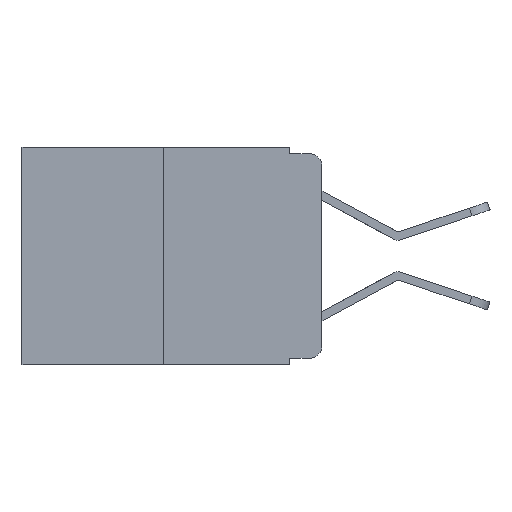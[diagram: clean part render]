
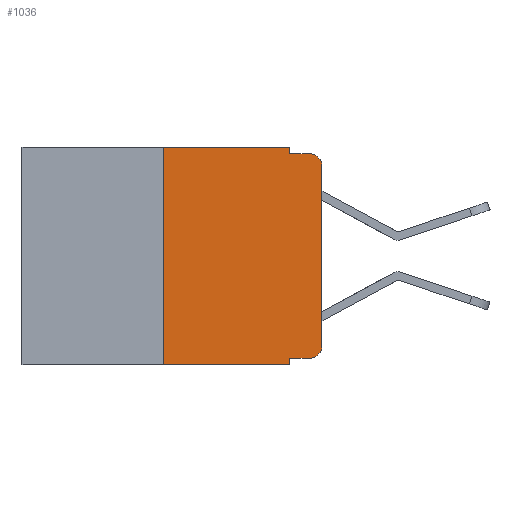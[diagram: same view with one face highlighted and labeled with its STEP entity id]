
A CAD part, left-side view. The second image highlights one B-rep face of the part: STEP entity #1036.
In plain terms, the highlighted planar face has unit normal (-1, 0, 0).
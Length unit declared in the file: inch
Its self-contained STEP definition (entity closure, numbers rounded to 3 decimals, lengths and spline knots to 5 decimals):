
#173 = VECTOR ( 'NONE', #9274, 39.37008 ) ;
#390 = DIRECTION ( 'NONE',  ( 0., 0., 1. ) ) ;
#671 = ORIENTED_EDGE ( 'NONE', *, *, #6945, .F. ) ;
#706 = ORIENTED_EDGE ( 'NONE', *, *, #1145, .T. ) ;
#812 = VERTEX_POINT ( 'NONE', #8968 ) ;
#838 = VECTOR ( 'NONE', #9036, 39.37008 ) ;
#891 = AXIS2_PLACEMENT_3D ( 'NONE', #4014, #6603, #8453 ) ;
#997 = EDGE_CURVE ( 'NONE', #5540, #1076, #4803, .T. ) ;
#1036 = ADVANCED_FACE ( 'NONE', ( #9545 ), #1417, .F. ) ;
#1076 = VERTEX_POINT ( 'NONE', #3899 ) ;
#1145 = EDGE_CURVE ( 'NONE', #6084, #10021, #8839, .T. ) ;
#1417 = PLANE ( 'NONE',  #11151 ) ;
#1558 = CIRCLE ( 'NONE', #891, 0.02 ) ;
#1885 = VECTOR ( 'NONE', #390, 39.37008 ) ;
#2099 = DIRECTION ( 'NONE',  ( 0., 0., -1. ) ) ;
#2164 = CARTESIAN_POINT ( 'NONE',  ( 0., 0.25, -0.343 ) ) ;
#2436 = VECTOR ( 'NONE', #10872, 39.37008 ) ;
#2442 = ORIENTED_EDGE ( 'NONE', *, *, #4425, .T. ) ;
#2454 = LINE ( 'NONE', #2854, #6899 ) ;
#2483 = EDGE_CURVE ( 'NONE', #10021, #6501, #1558, .T. ) ;
#2607 = VECTOR ( 'NONE', #9670, 39.37008 ) ;
#2854 = CARTESIAN_POINT ( 'NONE',  ( 0., 0.473, -0.343 ) ) ;
#3284 = CARTESIAN_POINT ( 'NONE',  ( 0., 0., -0.03 ) ) ;
#3309 = ORIENTED_EDGE ( 'NONE', *, *, #2483, .T. ) ;
#3342 = VECTOR ( 'NONE', #6471, 39.37008 ) ;
#3740 = CARTESIAN_POINT ( 'NONE',  ( 0., 0.25, 0. ) ) ;
#3899 = CARTESIAN_POINT ( 'NONE',  ( 0., 0.051, -0.01 ) ) ;
#3962 = CARTESIAN_POINT ( 'NONE',  ( 0., 0.051, 0. ) ) ;
#4012 = AXIS2_PLACEMENT_3D ( 'NONE', #4863, #10195, #11052 ) ;
#4014 = CARTESIAN_POINT ( 'NONE',  ( 0., 0.02, -0.313 ) ) ;
#4425 = EDGE_CURVE ( 'NONE', #6501, #5784, #9915, .T. ) ;
#4803 = LINE ( 'NONE', #5605, #2436 ) ;
#4863 = CARTESIAN_POINT ( 'NONE',  ( 0., 0.02, -0.03 ) ) ;
#4910 = CARTESIAN_POINT ( 'NONE',  ( 0., 0., 0. ) ) ;
#4959 = ORIENTED_EDGE ( 'NONE', *, *, #7851, .T. ) ;
#5017 = CARTESIAN_POINT ( 'NONE',  ( 0., 0.051, -0.343 ) ) ;
#5230 = CARTESIAN_POINT ( 'NONE',  ( 0., 0.02, -0.01 ) ) ;
#5472 = EDGE_CURVE ( 'NONE', #5784, #6966, #6820, .T. ) ;
#5531 = VERTEX_POINT ( 'NONE', #2164 ) ;
#5540 = VERTEX_POINT ( 'NONE', #3962 ) ;
#5546 = EDGE_CURVE ( 'NONE', #1076, #6966, #10741, .T. ) ;
#5605 = CARTESIAN_POINT ( 'NONE',  ( 0., 0.051, 0. ) ) ;
#5784 = VERTEX_POINT ( 'NONE', #3284 ) ;
#5953 = LINE ( 'NONE', #7945, #2607 ) ;
#6084 = VERTEX_POINT ( 'NONE', #10963 ) ;
#6452 = DIRECTION ( 'NONE',  ( 0., -1., 0. ) ) ;
#6471 = DIRECTION ( 'NONE',  ( 0., -1., 0. ) ) ;
#6501 = VERTEX_POINT ( 'NONE', #7286 ) ;
#6603 = DIRECTION ( 'NONE',  ( -1., 0., 0. ) ) ;
#6605 = DIRECTION ( 'NONE',  ( 1., 0., 0. ) ) ;
#6758 = DIRECTION ( 'NONE',  ( 0., -1., 0. ) ) ;
#6820 = CIRCLE ( 'NONE', #4012, 0.02 ) ;
#6899 = VECTOR ( 'NONE', #6452, 39.37008 ) ;
#6945 = EDGE_CURVE ( 'NONE', #6084, #7473, #5953, .T. ) ;
#6966 = VERTEX_POINT ( 'NONE', #5230 ) ;
#7145 = EDGE_CURVE ( 'NONE', #812, #5540, #7334, .T. ) ;
#7286 = CARTESIAN_POINT ( 'NONE',  ( 0., 0., -0.313 ) ) ;
#7296 = ORIENTED_EDGE ( 'NONE', *, *, #5472, .T. ) ;
#7334 = LINE ( 'NONE', #8100, #838 ) ;
#7473 = VERTEX_POINT ( 'NONE', #5017 ) ;
#7668 = CARTESIAN_POINT ( 'NONE',  ( 0., 0.051, -0.333 ) ) ;
#7851 = EDGE_CURVE ( 'NONE', #5531, #7473, #2454, .T. ) ;
#7870 = EDGE_CURVE ( 'NONE', #5531, #812, #9003, .T. ) ;
#7945 = CARTESIAN_POINT ( 'NONE',  ( 0., 0.051, 0. ) ) ;
#8100 = CARTESIAN_POINT ( 'NONE',  ( 0., 0.473, 0. ) ) ;
#8308 = ORIENTED_EDGE ( 'NONE', *, *, #7145, .F. ) ;
#8453 = DIRECTION ( 'NONE',  ( 0., 0., -1. ) ) ;
#8753 = ORIENTED_EDGE ( 'NONE', *, *, #7870, .F. ) ;
#8839 = LINE ( 'NONE', #7668, #11208 ) ;
#8968 = CARTESIAN_POINT ( 'NONE',  ( 0., 0.25, 0. ) ) ;
#9003 = LINE ( 'NONE', #3740, #1885 ) ;
#9007 = CARTESIAN_POINT ( 'NONE',  ( 0., 0.02, -0.333 ) ) ;
#9036 = DIRECTION ( 'NONE',  ( 0., -1., 0. ) ) ;
#9190 = CARTESIAN_POINT ( 'NONE',  ( 0., 0.051, -0.01 ) ) ;
#9274 = DIRECTION ( 'NONE',  ( 0., 0., 1. ) ) ;
#9366 = CARTESIAN_POINT ( 'NONE',  ( 0., 0.473, 0. ) ) ;
#9545 = FACE_OUTER_BOUND ( 'NONE', #10308, .T. ) ;
#9612 = ORIENTED_EDGE ( 'NONE', *, *, #997, .F. ) ;
#9670 = DIRECTION ( 'NONE',  ( 0., 0., -1. ) ) ;
#9915 = LINE ( 'NONE', #4910, #173 ) ;
#10021 = VERTEX_POINT ( 'NONE', #9007 ) ;
#10195 = DIRECTION ( 'NONE',  ( -1., 0., 0. ) ) ;
#10308 = EDGE_LOOP ( 'NONE', ( #2442, #7296, #10853, #9612, #8308, #8753, #4959, #671, #706, #3309 ) ) ;
#10741 = LINE ( 'NONE', #9190, #3342 ) ;
#10853 = ORIENTED_EDGE ( 'NONE', *, *, #5546, .F. ) ;
#10872 = DIRECTION ( 'NONE',  ( 0., 0., -1. ) ) ;
#10963 = CARTESIAN_POINT ( 'NONE',  ( 0., 0.051, -0.333 ) ) ;
#11052 = DIRECTION ( 'NONE',  ( 0., 0., -1. ) ) ;
#11151 = AXIS2_PLACEMENT_3D ( 'NONE', #9366, #6605, #2099 ) ;
#11208 = VECTOR ( 'NONE', #6758, 39.37008 ) ;
